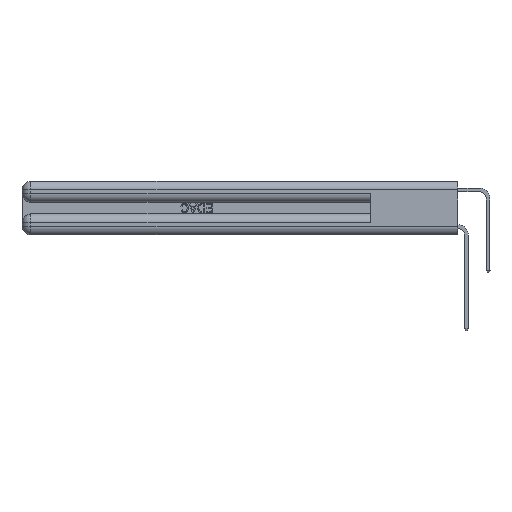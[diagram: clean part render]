
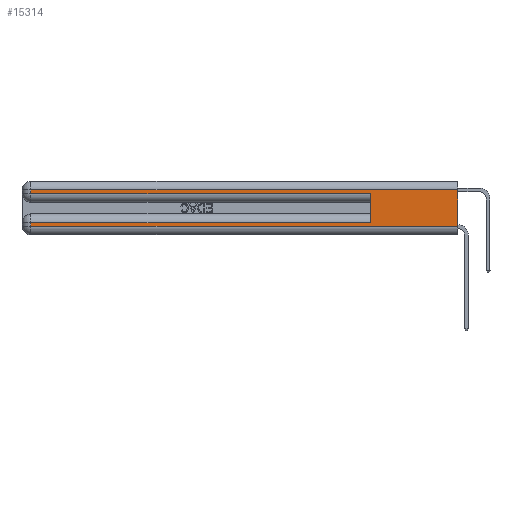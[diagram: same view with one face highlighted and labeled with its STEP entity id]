
A CAD part, left-side view. The second image highlights one B-rep face of the part: STEP entity #15314.
In plain terms, the highlighted planar face has unit normal (-1, 0, 0).
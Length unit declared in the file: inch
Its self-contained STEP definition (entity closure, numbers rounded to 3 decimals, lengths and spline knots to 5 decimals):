
#555 = ORIENTED_EDGE ( 'NONE', *, *, #11861, .T. ) ;
#651 = CARTESIAN_POINT ( 'NONE',  ( 0., 0.6, 0.085 ) ) ;
#1295 = CARTESIAN_POINT ( 'NONE',  ( 0., 2.94, 0.085 ) ) ;
#1870 = EDGE_CURVE ( 'NONE', #6902, #10617, #25701, .T. ) ;
#2140 = EDGE_CURVE ( 'NONE', #24218, #13614, #32472, .T. ) ;
#3157 = ORIENTED_EDGE ( 'NONE', *, *, #26826, .T. ) ;
#3603 = VECTOR ( 'NONE', #27429, 39.37008 ) ;
#3950 = EDGE_CURVE ( 'NONE', #29219, #24218, #26392, .T. ) ;
#4415 = DIRECTION ( 'NONE',  ( 0., 0., -1. ) ) ;
#4843 = CARTESIAN_POINT ( 'NONE',  ( 0., 2.94, 0.37 ) ) ;
#5210 = ORIENTED_EDGE ( 'NONE', *, *, #6855, .T. ) ;
#6604 = CARTESIAN_POINT ( 'NONE',  ( 0., 0., 0.06 ) ) ;
#6855 = EDGE_CURVE ( 'NONE', #28842, #29219, #11824, .T. ) ;
#6902 = VERTEX_POINT ( 'NONE', #28662 ) ;
#7435 = DIRECTION ( 'NONE',  ( 0., 0., -1. ) ) ;
#7516 = CARTESIAN_POINT ( 'NONE',  ( 0., 0.6, 0.145 ) ) ;
#9246 = CARTESIAN_POINT ( 'NONE',  ( 0., 2.94, 0.285 ) ) ;
#9855 = VECTOR ( 'NONE', #14595, 39.37008 ) ;
#9949 = VERTEX_POINT ( 'NONE', #23892 ) ;
#10617 = VERTEX_POINT ( 'NONE', #9246 ) ;
#11824 = LINE ( 'NONE', #32860, #9855 ) ;
#11861 = EDGE_CURVE ( 'NONE', #10617, #9949, #33070, .T. ) ;
#12318 = CARTESIAN_POINT ( 'NONE',  ( 0., 2.94, 0.37 ) ) ;
#13614 = VERTEX_POINT ( 'NONE', #6604 ) ;
#14462 = DIRECTION ( 'NONE',  ( 0., -1., 0. ) ) ;
#14595 = DIRECTION ( 'NONE',  ( 0., 1., 0. ) ) ;
#14633 = CARTESIAN_POINT ( 'NONE',  ( 0., 0., 0.285 ) ) ;
#15169 = ORIENTED_EDGE ( 'NONE', *, *, #3950, .T. ) ;
#15303 = CARTESIAN_POINT ( 'NONE',  ( 0., 2.94, 0.06 ) ) ;
#15314 = ADVANCED_FACE ( 'NONE', ( #19721 ), #32753, .F. ) ;
#15521 = DIRECTION ( 'NONE',  ( 0., 0., 1. ) ) ;
#15802 = VECTOR ( 'NONE', #17711, 39.37008 ) ;
#15978 = ORIENTED_EDGE ( 'NONE', *, *, #32309, .F. ) ;
#16482 = CARTESIAN_POINT ( 'NONE',  ( 0., 0., 0.06 ) ) ;
#16692 = VECTOR ( 'NONE', #18527, 39.37008 ) ;
#17711 = DIRECTION ( 'NONE',  ( 0., 0., -1. ) ) ;
#18313 = VECTOR ( 'NONE', #14462, 39.37008 ) ;
#18380 = AXIS2_PLACEMENT_3D ( 'NONE', #27547, #25096, #30138 ) ;
#18527 = DIRECTION ( 'NONE',  ( 0., 1., 0. ) ) ;
#18766 = VECTOR ( 'NONE', #7435, 39.37008 ) ;
#19721 = FACE_OUTER_BOUND ( 'NONE', #30038, .T. ) ;
#23432 = ORIENTED_EDGE ( 'NONE', *, *, #32503, .F. ) ;
#23892 = CARTESIAN_POINT ( 'NONE',  ( 0., 0.6, 0.285 ) ) ;
#24218 = VERTEX_POINT ( 'NONE', #15303 ) ;
#25096 = DIRECTION ( 'NONE',  ( 1., 0., 0. ) ) ;
#25701 = LINE ( 'NONE', #12318, #15802 ) ;
#26120 = LINE ( 'NONE', #7516, #31844 ) ;
#26392 = LINE ( 'NONE', #4843, #18766 ) ;
#26618 = VERTEX_POINT ( 'NONE', #30193 ) ;
#26826 = EDGE_CURVE ( 'NONE', #26618, #6902, #28782, .T. ) ;
#27429 = DIRECTION ( 'NONE',  ( 0., -1., 0. ) ) ;
#27547 = CARTESIAN_POINT ( 'NONE',  ( 0., 0., 0.37 ) ) ;
#28662 = CARTESIAN_POINT ( 'NONE',  ( 0., 2.94, 0.31 ) ) ;
#28782 = LINE ( 'NONE', #28951, #16692 ) ;
#28842 = VERTEX_POINT ( 'NONE', #651 ) ;
#28951 = CARTESIAN_POINT ( 'NONE',  ( 0., 0., 0.31 ) ) ;
#29219 = VERTEX_POINT ( 'NONE', #1295 ) ;
#29833 = CARTESIAN_POINT ( 'NONE',  ( 0., 0., 0.37 ) ) ;
#30038 = EDGE_LOOP ( 'NONE', ( #15978, #3157, #33031, #555, #23432, #5210, #15169, #33580 ) ) ;
#30138 = DIRECTION ( 'NONE',  ( 0., 0., -1. ) ) ;
#30193 = CARTESIAN_POINT ( 'NONE',  ( 0., 0., 0.31 ) ) ;
#30353 = LINE ( 'NONE', #29833, #32412 ) ;
#31844 = VECTOR ( 'NONE', #15521, 39.37008 ) ;
#32309 = EDGE_CURVE ( 'NONE', #26618, #13614, #30353, .T. ) ;
#32412 = VECTOR ( 'NONE', #4415, 39.37008 ) ;
#32472 = LINE ( 'NONE', #16482, #3603 ) ;
#32503 = EDGE_CURVE ( 'NONE', #28842, #9949, #26120, .T. ) ;
#32753 = PLANE ( 'NONE',  #18380 ) ;
#32860 = CARTESIAN_POINT ( 'NONE',  ( 0., 0., 0.085 ) ) ;
#33031 = ORIENTED_EDGE ( 'NONE', *, *, #1870, .T. ) ;
#33070 = LINE ( 'NONE', #14633, #18313 ) ;
#33580 = ORIENTED_EDGE ( 'NONE', *, *, #2140, .T. ) ;
